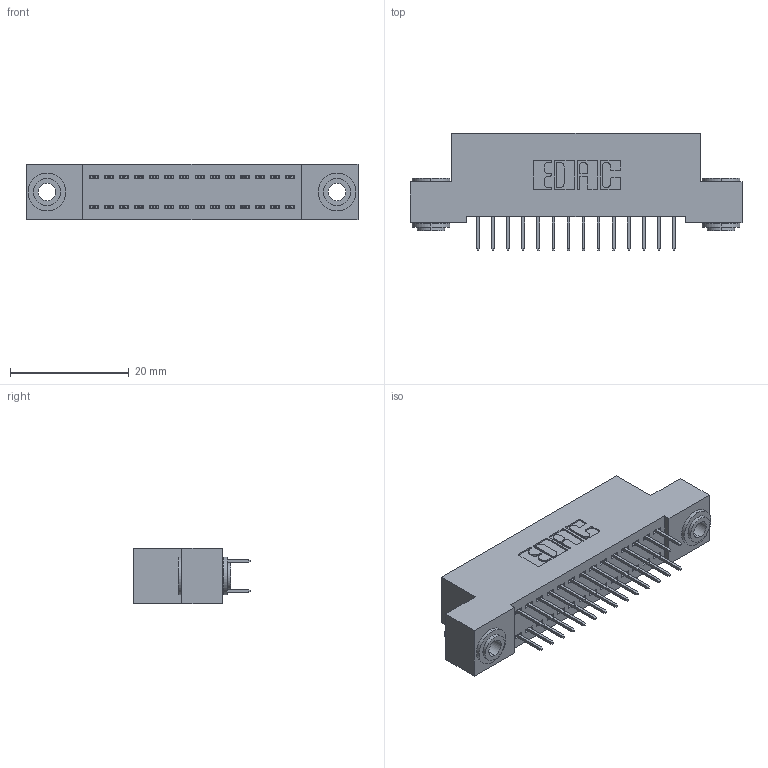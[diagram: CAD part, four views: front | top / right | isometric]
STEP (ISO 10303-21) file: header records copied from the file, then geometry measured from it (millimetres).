
FILE_DESCRIPTION (( 'STEP AP203' ), '1' );
FILE_NAME ('342-028-524-203.STEP', '2018-08-11T06:40:08', ( '' ), ( '' ), 'SwSTEP 2.0', 'SolidWorks 2016', '' );
FILE_SCHEMA (( 'CONFIG_CONTROL_DESIGN' ));
Length unit declared in the file: inch
Products named in the file (4): 345-292-001_345-293-124; 342-250-002_345-250-002-102; 342-028-524-203; 342 Part_.156 TH
Assembly tree (31 placements, depth 2):
  342-028-524-203
    342 Part_.156 TH
    345-292-001_345-293-124  x28
    342-250-002_345-250-002-102  x2
Bounding box: 55.88 x 19.69 x 9.4 mm (x, y, z)
Volume: 4868.7 mm3; surface area: 7339 mm2
Topology: 31 solids, 31 shells, 1716 faces, 4827 edges, 3102 vertices
Faces by surface type: plane 1252, cylinder 456, cone 8
Entity records: 13220 total; most frequent: CARTESIAN_POINT 2197, ORIENTED_EDGE 2126, DIRECTION 1961, EDGE_CURVE 1063, LINE 915, VECTOR 915, VERTEX_POINT 702, AXIS2_PLACEMENT_3D 523
